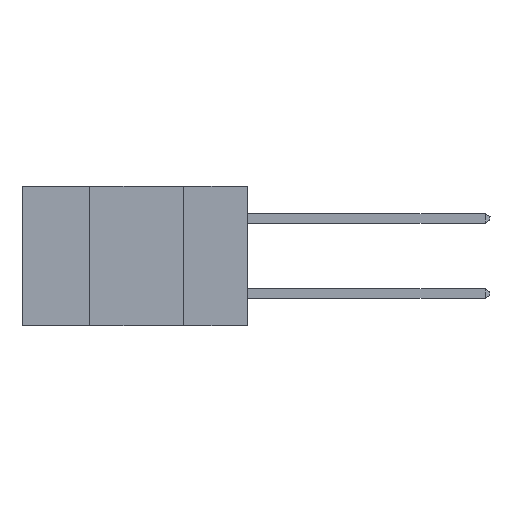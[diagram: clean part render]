
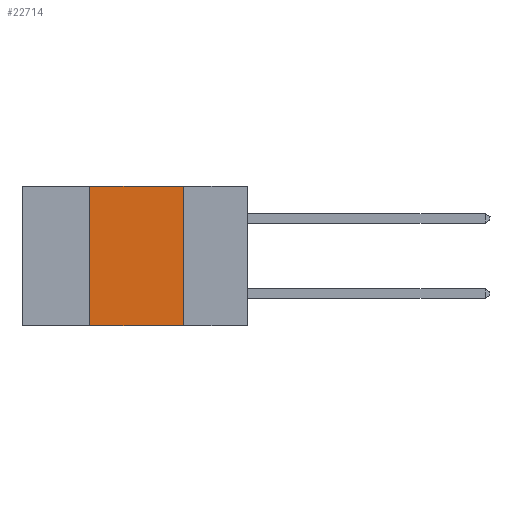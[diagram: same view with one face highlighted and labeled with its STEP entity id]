
A CAD part, left-side view. The second image highlights one B-rep face of the part: STEP entity #22714.
In plain terms, the highlighted planar face has unit normal (-1, 0, 0).
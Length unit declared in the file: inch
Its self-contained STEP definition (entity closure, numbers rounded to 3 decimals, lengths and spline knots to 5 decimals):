
#1133 = CARTESIAN_POINT ( 'NONE',  ( 0., 0.42, 0. ) ) ;
#3162 = DIRECTION ( 'NONE',  ( 0., -1., 0. ) ) ;
#3601 = ORIENTED_EDGE ( 'NONE', *, *, #23283, .T. ) ;
#3605 = DIRECTION ( 'NONE',  ( 0., 0., -1. ) ) ;
#4306 = VECTOR ( 'NONE', #3605, 39.37008 ) ;
#5020 = ORIENTED_EDGE ( 'NONE', *, *, #25254, .F. ) ;
#5892 = EDGE_CURVE ( 'NONE', #9880, #22680, #18948, .T. ) ;
#6290 = AXIS2_PLACEMENT_3D ( 'NONE', #18486, #23548, #20978 ) ;
#6334 = VECTOR ( 'NONE', #3162, 39.37008 ) ;
#6464 = EDGE_LOOP ( 'NONE', ( #15519, #20002, #5020, #3601 ) ) ;
#7581 = CARTESIAN_POINT ( 'NONE',  ( 0., 0.42, -0.37 ) ) ;
#9147 = PLANE ( 'NONE',  #6290 ) ;
#9691 = VECTOR ( 'NONE', #28439, 39.37008 ) ;
#9880 = VERTEX_POINT ( 'NONE', #19944 ) ;
#10836 = CARTESIAN_POINT ( 'NONE',  ( 0., 0.17, -0.37 ) ) ;
#11552 = CARTESIAN_POINT ( 'NONE',  ( 0., 0.17, 0. ) ) ;
#11597 = FACE_OUTER_BOUND ( 'NONE', #6464, .T. ) ;
#14459 = VERTEX_POINT ( 'NONE', #10836 ) ;
#15519 = ORIENTED_EDGE ( 'NONE', *, *, #19145, .F. ) ;
#15922 = VECTOR ( 'NONE', #24838, 39.37008 ) ;
#17056 = CARTESIAN_POINT ( 'NONE',  ( 0., 0.6, 0. ) ) ;
#17476 = LINE ( 'NONE', #18987, #9691 ) ;
#18486 = CARTESIAN_POINT ( 'NONE',  ( 0., 0.6, 0. ) ) ;
#18948 = LINE ( 'NONE', #17056, #6334 ) ;
#18987 = CARTESIAN_POINT ( 'NONE',  ( 0., 0.6, -0.37 ) ) ;
#19145 = EDGE_CURVE ( 'NONE', #22680, #14459, #21752, .T. ) ;
#19944 = CARTESIAN_POINT ( 'NONE',  ( 0., 0.42, 0. ) ) ;
#20002 = ORIENTED_EDGE ( 'NONE', *, *, #5892, .F. ) ;
#20978 = DIRECTION ( 'NONE',  ( 0., 0., -1. ) ) ;
#20994 = VERTEX_POINT ( 'NONE', #7581 ) ;
#21752 = LINE ( 'NONE', #22289, #4306 ) ;
#22289 = CARTESIAN_POINT ( 'NONE',  ( 0., 0.17, 0. ) ) ;
#22680 = VERTEX_POINT ( 'NONE', #11552 ) ;
#22714 = ADVANCED_FACE ( 'NONE', ( #11597 ), #9147, .F. ) ;
#23283 = EDGE_CURVE ( 'NONE', #20994, #14459, #17476, .T. ) ;
#23548 = DIRECTION ( 'NONE',  ( 1., 0., 0. ) ) ;
#24838 = DIRECTION ( 'NONE',  ( 0., 0., 1. ) ) ;
#25254 = EDGE_CURVE ( 'NONE', #20994, #9880, #26284, .T. ) ;
#26284 = LINE ( 'NONE', #1133, #15922 ) ;
#28439 = DIRECTION ( 'NONE',  ( 0., -1., 0. ) ) ;
